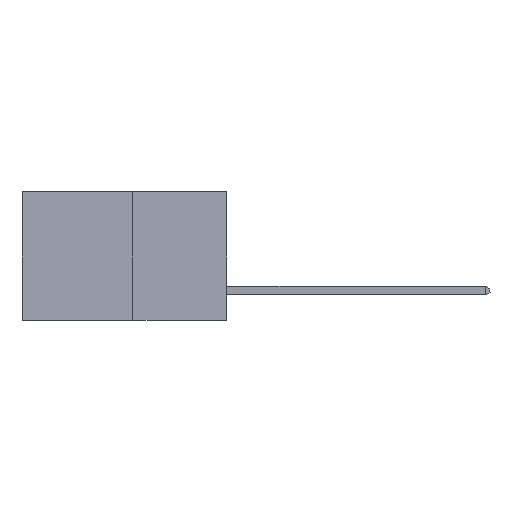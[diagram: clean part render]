
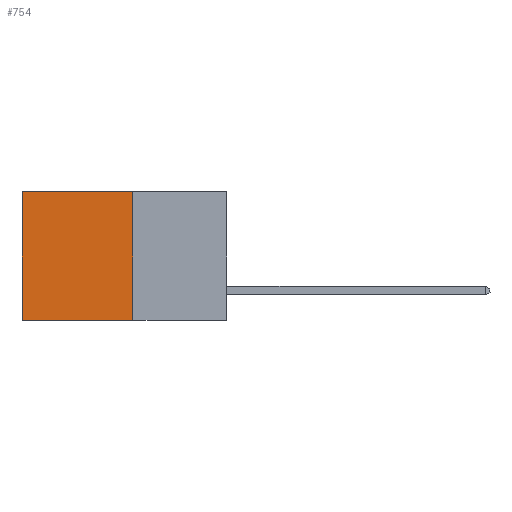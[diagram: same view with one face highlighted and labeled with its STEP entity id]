
A CAD part, left-side view. The second image highlights one B-rep face of the part: STEP entity #754.
In plain terms, the highlighted planar face has unit normal (-1, 0, 0).
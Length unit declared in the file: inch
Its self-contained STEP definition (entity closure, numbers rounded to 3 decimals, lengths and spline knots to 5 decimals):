
#619 = ORIENTED_EDGE ( 'NONE', *, *, #6746, .T. ) ;
#754 = ADVANCED_FACE ( 'NONE', ( #2704 ), #10032, .F. ) ;
#2436 = EDGE_LOOP ( 'NONE', ( #2821, #8344, #11349, #619 ) ) ;
#2704 = FACE_OUTER_BOUND ( 'NONE', #2436, .T. ) ;
#2821 = ORIENTED_EDGE ( 'NONE', *, *, #5127, .T. ) ;
#3413 = VECTOR ( 'NONE', #12364, 39.37008 ) ;
#3786 = CARTESIAN_POINT ( 'NONE',  ( 0.277, 0.59, -0.37 ) ) ;
#3894 = LINE ( 'NONE', #6444, #11135 ) ;
#4172 = CARTESIAN_POINT ( 'NONE',  ( 0.277, 0.27, -0.37 ) ) ;
#4186 = AXIS2_PLACEMENT_3D ( 'NONE', #11027, #11707, #12961 ) ;
#4243 = VERTEX_POINT ( 'NONE', #11538 ) ;
#4344 = LINE ( 'NONE', #6939, #9509 ) ;
#5127 = EDGE_CURVE ( 'NONE', #4243, #11832, #3894, .T. ) ;
#5852 = DIRECTION ( 'NONE',  ( 0., 1., 0. ) ) ;
#6444 = CARTESIAN_POINT ( 'NONE',  ( 0.277, 0.59, -0.37 ) ) ;
#6746 = EDGE_CURVE ( 'NONE', #12071, #4243, #4344, .T. ) ;
#6939 = CARTESIAN_POINT ( 'NONE',  ( 0.277, 0.27, 0. ) ) ;
#7481 = DIRECTION ( 'NONE',  ( 0., 0., -1. ) ) ;
#8109 = EDGE_CURVE ( 'NONE', #10798, #11832, #8853, .T. ) ;
#8319 = CARTESIAN_POINT ( 'NONE',  ( 0.277, 0.27, 0. ) ) ;
#8344 = ORIENTED_EDGE ( 'NONE', *, *, #8109, .F. ) ;
#8853 = LINE ( 'NONE', #10552, #9162 ) ;
#9162 = VECTOR ( 'NONE', #11559, 39.37008 ) ;
#9492 = CARTESIAN_POINT ( 'NONE',  ( 0.277, 0.27, -0.37 ) ) ;
#9509 = VECTOR ( 'NONE', #5852, 39.37008 ) ;
#10032 = PLANE ( 'NONE',  #4186 ) ;
#10552 = CARTESIAN_POINT ( 'NONE',  ( 0.277, 0.27, -0.37 ) ) ;
#10705 = EDGE_CURVE ( 'NONE', #12071, #10798, #11914, .T. ) ;
#10798 = VERTEX_POINT ( 'NONE', #9492 ) ;
#11027 = CARTESIAN_POINT ( 'NONE',  ( 0.277, 0.27, -0.37 ) ) ;
#11135 = VECTOR ( 'NONE', #7481, 39.37008 ) ;
#11349 = ORIENTED_EDGE ( 'NONE', *, *, #10705, .F. ) ;
#11538 = CARTESIAN_POINT ( 'NONE',  ( 0.277, 0.59, 0. ) ) ;
#11559 = DIRECTION ( 'NONE',  ( 0., 1., 0. ) ) ;
#11707 = DIRECTION ( 'NONE',  ( 1., 0., 0. ) ) ;
#11832 = VERTEX_POINT ( 'NONE', #3786 ) ;
#11914 = LINE ( 'NONE', #4172, #3413 ) ;
#12071 = VERTEX_POINT ( 'NONE', #8319 ) ;
#12364 = DIRECTION ( 'NONE',  ( 0., 0., -1. ) ) ;
#12961 = DIRECTION ( 'NONE',  ( 0., 0., -1. ) ) ;
